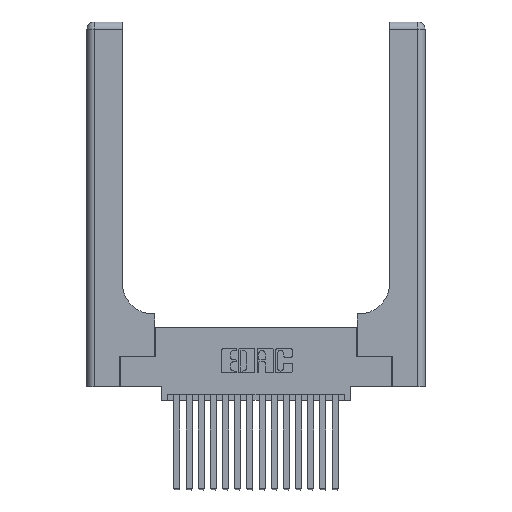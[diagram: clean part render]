
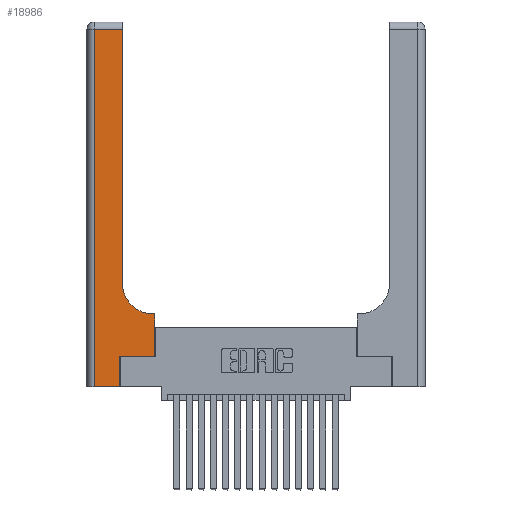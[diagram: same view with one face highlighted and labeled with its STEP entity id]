
A CAD part, top view. The second image highlights one B-rep face of the part: STEP entity #18986.
In plain terms, the highlighted planar face has unit normal (0, 0, 1).
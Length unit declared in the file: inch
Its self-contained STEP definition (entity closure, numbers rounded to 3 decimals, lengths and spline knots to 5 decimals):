
#380 = CARTESIAN_POINT ( 'NONE',  ( 0., 3., 0.37 ) ) ;
#516 = VERTEX_POINT ( 'NONE', #15680 ) ;
#547 = LINE ( 'NONE', #10083, #12481 ) ;
#717 = DIRECTION ( 'NONE',  ( 1., 0., 0. ) ) ;
#789 = DIRECTION ( 'NONE',  ( -1., 0., 0. ) ) ;
#1526 = LINE ( 'NONE', #19124, #9773 ) ;
#1619 = CARTESIAN_POINT ( 'NONE',  ( 0.5415, 0.85, 0.37 ) ) ;
#1955 = DIRECTION ( 'NONE',  ( -1., 0., 0. ) ) ;
#2040 = AXIS2_PLACEMENT_3D ( 'NONE', #1619, #12505, #3204 ) ;
#2163 = VECTOR ( 'NONE', #17120, 39.37008 ) ;
#2197 = VERTEX_POINT ( 'NONE', #15997 ) ;
#2603 = EDGE_CURVE ( 'NONE', #10164, #15190, #14765, .T. ) ;
#3204 = DIRECTION ( 'NONE',  ( 1., 0., 0. ) ) ;
#3544 = EDGE_CURVE ( 'NONE', #4213, #10885, #4106, .T. ) ;
#3647 = CARTESIAN_POINT ( 'NONE',  ( 0.06, 3., 0.37 ) ) ;
#4106 = LINE ( 'NONE', #3647, #19886 ) ;
#4157 = DIRECTION ( 'NONE',  ( -1., 0., 0. ) ) ;
#4213 = VERTEX_POINT ( 'NONE', #13048 ) ;
#4575 = EDGE_LOOP ( 'NONE', ( #9054, #10091, #8074, #15655, #11336, #15114, #6380, #10185, #7651 ) ) ;
#4644 = EDGE_CURVE ( 'NONE', #10885, #13147, #10913, .T. ) ;
#4664 = EDGE_CURVE ( 'NONE', #516, #2197, #18505, .T. ) ;
#6202 = CARTESIAN_POINT ( 'NONE',  ( 0.269, 0., 0.37 ) ) ;
#6278 = VECTOR ( 'NONE', #17052, 39.37008 ) ;
#6380 = ORIENTED_EDGE ( 'NONE', *, *, #2603, .T. ) ;
#7170 = CARTESIAN_POINT ( 'NONE',  ( 0.2915, 0.6, 0.37 ) ) ;
#7277 = LINE ( 'NONE', #7170, #10935 ) ;
#7351 = CARTESIAN_POINT ( 'NONE',  ( 0.5415, 0.6, 0.37 ) ) ;
#7415 = CARTESIAN_POINT ( 'NONE',  ( 0.06, 0., 0.37 ) ) ;
#7651 = ORIENTED_EDGE ( 'NONE', *, *, #18824, .T. ) ;
#7855 = CARTESIAN_POINT ( 'NONE',  ( 0., 0., 0.37 ) ) ;
#8074 = ORIENTED_EDGE ( 'NONE', *, *, #3544, .T. ) ;
#8719 = DIRECTION ( 'NONE',  ( 0., 1., 0. ) ) ;
#8723 = CARTESIAN_POINT ( 'NONE',  ( 0.5585, 0.25, 0.37 ) ) ;
#9054 = ORIENTED_EDGE ( 'NONE', *, *, #4664, .T. ) ;
#9412 = CARTESIAN_POINT ( 'NONE',  ( 0.2915, 3., 0.37 ) ) ;
#9773 = VECTOR ( 'NONE', #717, 39.37008 ) ;
#10083 = CARTESIAN_POINT ( 'NONE',  ( 0.269, 0., 0.37 ) ) ;
#10091 = ORIENTED_EDGE ( 'NONE', *, *, #18094, .T. ) ;
#10141 = EDGE_CURVE ( 'NONE', #15190, #10844, #7277, .T. ) ;
#10150 = DIRECTION ( 'NONE',  ( 0., 1., 0. ) ) ;
#10164 = VERTEX_POINT ( 'NONE', #17961 ) ;
#10185 = ORIENTED_EDGE ( 'NONE', *, *, #10141, .T. ) ;
#10844 = VERTEX_POINT ( 'NONE', #7351 ) ;
#10885 = VERTEX_POINT ( 'NONE', #7415 ) ;
#10913 = LINE ( 'NONE', #7855, #6278 ) ;
#10935 = VECTOR ( 'NONE', #4157, 39.37008 ) ;
#11129 = PLANE ( 'NONE',  #18522 ) ;
#11263 = DIRECTION ( 'NONE',  ( 0., 0., -1. ) ) ;
#11336 = ORIENTED_EDGE ( 'NONE', *, *, #16888, .T. ) ;
#12174 = VERTEX_POINT ( 'NONE', #15843 ) ;
#12481 = VECTOR ( 'NONE', #10150, 39.37008 ) ;
#12505 = DIRECTION ( 'NONE',  ( 0., 0., -1. ) ) ;
#12700 = FACE_OUTER_BOUND ( 'NONE', #4575, .T. ) ;
#13048 = CARTESIAN_POINT ( 'NONE',  ( 0.06, 2.94, 0.37 ) ) ;
#13147 = VERTEX_POINT ( 'NONE', #6202 ) ;
#14765 = LINE ( 'NONE', #8723, #15222 ) ;
#14895 = VECTOR ( 'NONE', #789, 39.37008 ) ;
#15114 = ORIENTED_EDGE ( 'NONE', *, *, #16850, .T. ) ;
#15190 = VERTEX_POINT ( 'NONE', #16526 ) ;
#15222 = VECTOR ( 'NONE', #8719, 39.37008 ) ;
#15565 = CIRCLE ( 'NONE', #2040, 0.25 ) ;
#15655 = ORIENTED_EDGE ( 'NONE', *, *, #4644, .T. ) ;
#15680 = CARTESIAN_POINT ( 'NONE',  ( 0.2915, 0.85, 0.37 ) ) ;
#15843 = CARTESIAN_POINT ( 'NONE',  ( 0.269, 0.25, 0.37 ) ) ;
#15997 = CARTESIAN_POINT ( 'NONE',  ( 0.2915, 2.94, 0.37 ) ) ;
#16526 = CARTESIAN_POINT ( 'NONE',  ( 0.5585, 0.6, 0.37 ) ) ;
#16850 = EDGE_CURVE ( 'NONE', #12174, #10164, #1526, .T. ) ;
#16888 = EDGE_CURVE ( 'NONE', #13147, #12174, #547, .T. ) ;
#17052 = DIRECTION ( 'NONE',  ( 1., 0., 0. ) ) ;
#17120 = DIRECTION ( 'NONE',  ( 0., 1., 0. ) ) ;
#17961 = CARTESIAN_POINT ( 'NONE',  ( 0.5585, 0.25, 0.37 ) ) ;
#18094 = EDGE_CURVE ( 'NONE', #2197, #4213, #18847, .T. ) ;
#18505 = LINE ( 'NONE', #9412, #2163 ) ;
#18522 = AXIS2_PLACEMENT_3D ( 'NONE', #380, #11263, #1955 ) ;
#18824 = EDGE_CURVE ( 'NONE', #10844, #516, #15565, .T. ) ;
#18847 = LINE ( 'NONE', #19190, #14895 ) ;
#18978 = DIRECTION ( 'NONE',  ( 0., -1., 0. ) ) ;
#18986 = ADVANCED_FACE ( 'NONE', ( #12700 ), #11129, .F. ) ;
#19124 = CARTESIAN_POINT ( 'NONE',  ( 0.269, 0.25, 0.37 ) ) ;
#19190 = CARTESIAN_POINT ( 'NONE',  ( 0., 2.94, 0.37 ) ) ;
#19886 = VECTOR ( 'NONE', #18978, 39.37008 ) ;
